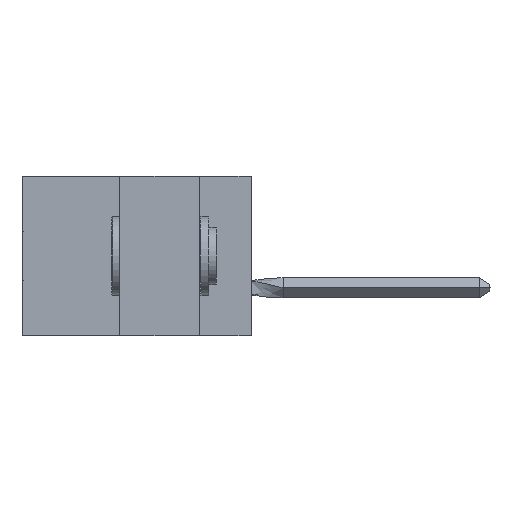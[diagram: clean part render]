
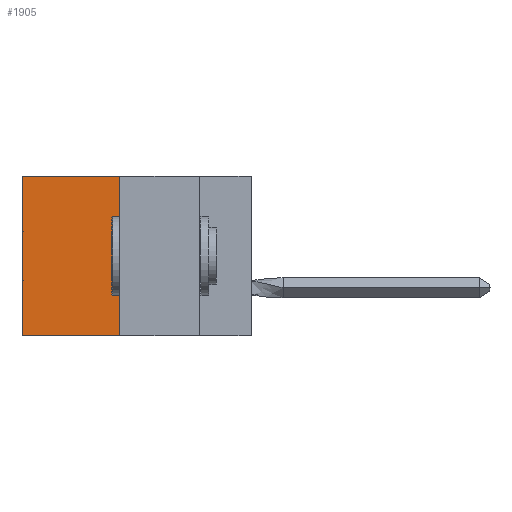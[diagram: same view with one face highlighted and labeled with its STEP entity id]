
A CAD part, left-side view. The second image highlights one B-rep face of the part: STEP entity #1905.
In plain terms, the highlighted planar face has unit normal (-1, 0, 0).
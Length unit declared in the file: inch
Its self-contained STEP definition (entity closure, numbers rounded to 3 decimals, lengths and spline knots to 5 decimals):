
#73 = DIRECTION ( 'NONE',  ( 0., 0., -1. ) ) ;
#1121 = ORIENTED_EDGE ( 'NONE', *, *, #11698, .T. ) ;
#1153 = CARTESIAN_POINT ( 'NONE',  ( 0.305, 0.72, -0.5 ) ) ;
#1160 = DIRECTION ( 'NONE',  ( 0., 1., 0. ) ) ;
#1461 = VECTOR ( 'NONE', #12389, 39.37008 ) ;
#1905 = ADVANCED_FACE ( 'NONE', ( #2664 ), #28625, .F. ) ;
#2664 = FACE_OUTER_BOUND ( 'NONE', #40519, .T. ) ;
#3978 = AXIS2_PLACEMENT_3D ( 'NONE', #12539, #41198, #73 ) ;
#4134 = LINE ( 'NONE', #6605, #17018 ) ;
#5092 = VERTEX_POINT ( 'NONE', #1153 ) ;
#5753 = EDGE_CURVE ( 'NONE', #7608, #12393, #30715, .T. ) ;
#6605 = CARTESIAN_POINT ( 'NONE',  ( 0.305, 0.413, -0.5 ) ) ;
#7608 = VERTEX_POINT ( 'NONE', #39953 ) ;
#8719 = EDGE_CURVE ( 'NONE', #12393, #5092, #4134, .T. ) ;
#11698 = EDGE_CURVE ( 'NONE', #40146, #5092, #35210, .T. ) ;
#12389 = DIRECTION ( 'NONE',  ( 0., 0., -1. ) ) ;
#12393 = VERTEX_POINT ( 'NONE', #40000 ) ;
#12539 = CARTESIAN_POINT ( 'NONE',  ( 0.305, 0.413, -0.5 ) ) ;
#12892 = CARTESIAN_POINT ( 'NONE',  ( 0.305, 0.413, 0. ) ) ;
#15256 = VECTOR ( 'NONE', #1160, 39.37008 ) ;
#15808 = VECTOR ( 'NONE', #39573, 39.37008 ) ;
#17018 = VECTOR ( 'NONE', #38413, 39.37008 ) ;
#18127 = ORIENTED_EDGE ( 'NONE', *, *, #5753, .F. ) ;
#23290 = CARTESIAN_POINT ( 'NONE',  ( 0.305, 0.72, -0.5 ) ) ;
#23708 = LINE ( 'NONE', #12892, #15256 ) ;
#24225 = ORIENTED_EDGE ( 'NONE', *, *, #8719, .F. ) ;
#28190 = CARTESIAN_POINT ( 'NONE',  ( 0.305, 0.413, -0.5 ) ) ;
#28625 = PLANE ( 'NONE',  #3978 ) ;
#30715 = LINE ( 'NONE', #28190, #1461 ) ;
#35210 = LINE ( 'NONE', #23290, #15808 ) ;
#35673 = CARTESIAN_POINT ( 'NONE',  ( 0.305, 0.72, 0. ) ) ;
#38413 = DIRECTION ( 'NONE',  ( 0., 1., 0. ) ) ;
#39573 = DIRECTION ( 'NONE',  ( 0., 0., -1. ) ) ;
#39953 = CARTESIAN_POINT ( 'NONE',  ( 0.305, 0.413, 0. ) ) ;
#40000 = CARTESIAN_POINT ( 'NONE',  ( 0.305, 0.413, -0.5 ) ) ;
#40146 = VERTEX_POINT ( 'NONE', #35673 ) ;
#40221 = EDGE_CURVE ( 'NONE', #7608, #40146, #23708, .T. ) ;
#40519 = EDGE_LOOP ( 'NONE', ( #1121, #24225, #18127, #40956 ) ) ;
#40956 = ORIENTED_EDGE ( 'NONE', *, *, #40221, .T. ) ;
#41198 = DIRECTION ( 'NONE',  ( 1., 0., 0. ) ) ;
